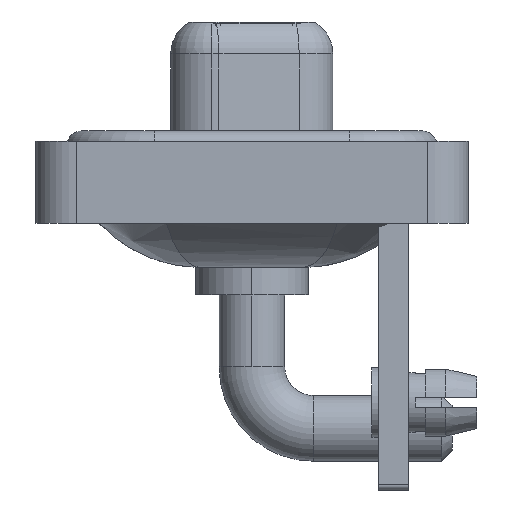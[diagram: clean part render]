
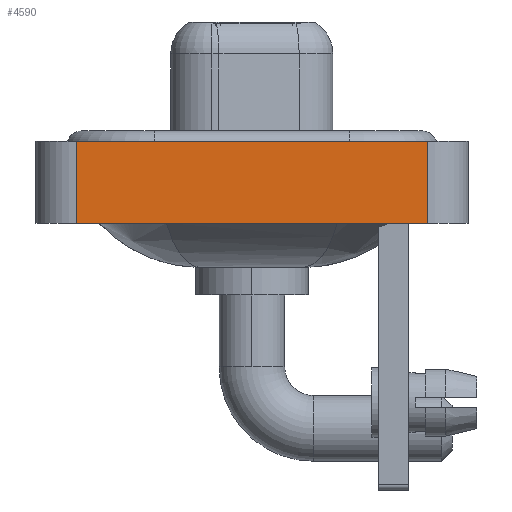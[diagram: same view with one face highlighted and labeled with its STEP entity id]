
A CAD part, left-side view. The second image highlights one B-rep face of the part: STEP entity #4590.
In plain terms, the highlighted planar face has unit normal (-1, 0, 0).
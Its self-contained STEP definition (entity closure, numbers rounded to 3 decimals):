
#146 = EDGE_CURVE ( 'NONE', #1484, #7447, #2184, .T. ) ;
#588 = VECTOR ( 'NONE', #17981, 1000. ) ;
#590 = DIRECTION ( 'NONE',  ( 0., -1., 0. ) ) ;
#668 = VECTOR ( 'NONE', #12846, 1000. ) ;
#785 = AXIS2_PLACEMENT_3D ( 'NONE', #17593, #16007, #7647 ) ;
#1484 = VERTEX_POINT ( 'NONE', #18525 ) ;
#2184 = LINE ( 'NONE', #17735, #14319 ) ;
#2643 = ORIENTED_EDGE ( 'NONE', *, *, #146, .T. ) ;
#3035 = ORIENTED_EDGE ( 'NONE', *, *, #4169, .F. ) ;
#4169 = EDGE_CURVE ( 'NONE', #1484, #13748, #10958, .T. ) ;
#4590 = ADVANCED_FACE ( 'NONE', ( #7558 ), #6162, .T. ) ;
#6162 = PLANE ( 'NONE',  #785 ) ;
#6537 = ORIENTED_EDGE ( 'NONE', *, *, #8432, .F. ) ;
#7447 = VERTEX_POINT ( 'NONE', #7912 ) ;
#7558 = FACE_OUTER_BOUND ( 'NONE', #12850, .T. ) ;
#7647 = DIRECTION ( 'NONE',  ( 0., 0., 1. ) ) ;
#7912 = CARTESIAN_POINT ( 'NONE',  ( -7.3, -8.55, -3.6 ) ) ;
#7936 = VECTOR ( 'NONE', #12459, 1000. ) ;
#8432 = EDGE_CURVE ( 'NONE', #13748, #8861, #16470, .T. ) ;
#8808 = LINE ( 'NONE', #10316, #668 ) ;
#8861 = VERTEX_POINT ( 'NONE', #17958 ) ;
#9642 = CARTESIAN_POINT ( 'NONE',  ( -7.3, 8.55, -3.6 ) ) ;
#10316 = CARTESIAN_POINT ( 'NONE',  ( -7.3, -8.55, -3.6 ) ) ;
#10820 = EDGE_CURVE ( 'NONE', #7447, #8861, #8808, .T. ) ;
#10958 = LINE ( 'NONE', #9642, #7936 ) ;
#12264 = CARTESIAN_POINT ( 'NONE',  ( -7.3, -8.55, 0.4 ) ) ;
#12459 = DIRECTION ( 'NONE',  ( 0., 0., 1. ) ) ;
#12846 = DIRECTION ( 'NONE',  ( 0., 0., 1. ) ) ;
#12850 = EDGE_LOOP ( 'NONE', ( #14114, #6537, #3035, #2643 ) ) ;
#13748 = VERTEX_POINT ( 'NONE', #17430 ) ;
#14114 = ORIENTED_EDGE ( 'NONE', *, *, #10820, .T. ) ;
#14319 = VECTOR ( 'NONE', #590, 1000. ) ;
#16007 = DIRECTION ( 'NONE',  ( -1., 0., 0. ) ) ;
#16470 = LINE ( 'NONE', #12264, #588 ) ;
#17430 = CARTESIAN_POINT ( 'NONE',  ( -7.3, 8.55, 0.4 ) ) ;
#17593 = CARTESIAN_POINT ( 'NONE',  ( -7.3, -8.55, -3.6 ) ) ;
#17735 = CARTESIAN_POINT ( 'NONE',  ( -7.3, -8.55, -3.6 ) ) ;
#17958 = CARTESIAN_POINT ( 'NONE',  ( -7.3, -8.55, 0.4 ) ) ;
#17981 = DIRECTION ( 'NONE',  ( 0., -1., 0. ) ) ;
#18525 = CARTESIAN_POINT ( 'NONE',  ( -7.3, 8.55, -3.6 ) ) ;
